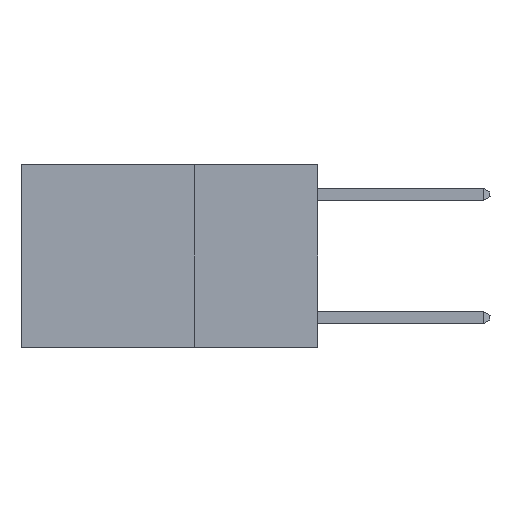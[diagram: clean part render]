
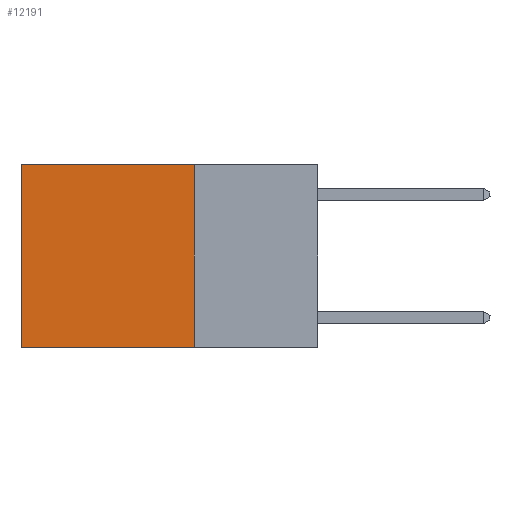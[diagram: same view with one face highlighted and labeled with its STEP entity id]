
A CAD part, left-side view. The second image highlights one B-rep face of the part: STEP entity #12191.
In plain terms, the highlighted planar face has unit normal (-1, 0, 0).
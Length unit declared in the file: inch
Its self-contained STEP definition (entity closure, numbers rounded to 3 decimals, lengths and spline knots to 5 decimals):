
#297 = EDGE_CURVE ( 'NONE', #19565, #20822, #7904, .T. ) ;
#400 = EDGE_CURVE ( 'NONE', #9023, #16624, #6276, .T. ) ;
#967 = DIRECTION ( 'NONE',  ( 0., 0., -1. ) ) ;
#1698 = ORIENTED_EDGE ( 'NONE', *, *, #400, .T. ) ;
#1816 = CARTESIAN_POINT ( 'NONE',  ( 0.2625, 0.25, 0. ) ) ;
#2086 = ORIENTED_EDGE ( 'NONE', *, *, #20383, .T. ) ;
#2225 = VECTOR ( 'NONE', #967, 39.37008 ) ;
#2647 = CARTESIAN_POINT ( 'NONE',  ( 0.2625, 0.6, 0. ) ) ;
#2873 = DIRECTION ( 'NONE',  ( 0., 0., -1. ) ) ;
#4243 = DIRECTION ( 'NONE',  ( 0., 0., -1. ) ) ;
#5708 = EDGE_LOOP ( 'NONE', ( #1698, #7116, #20183, #2086 ) ) ;
#6022 = AXIS2_PLACEMENT_3D ( 'NONE', #8006, #13166, #2873 ) ;
#6276 = LINE ( 'NONE', #2647, #2225 ) ;
#6412 = CARTESIAN_POINT ( 'NONE',  ( 0.2625, 0.25, -0.37 ) ) ;
#7116 = ORIENTED_EDGE ( 'NONE', *, *, #16803, .F. ) ;
#7751 = DIRECTION ( 'NONE',  ( 0., 1., 0. ) ) ;
#7904 = LINE ( 'NONE', #14473, #21235 ) ;
#8006 = CARTESIAN_POINT ( 'NONE',  ( 0.2625, 0.25, 0. ) ) ;
#9023 = VERTEX_POINT ( 'NONE', #10978 ) ;
#10761 = CARTESIAN_POINT ( 'NONE',  ( 0.2625, 0.6, -0.37 ) ) ;
#10978 = CARTESIAN_POINT ( 'NONE',  ( 0.2625, 0.6, 0. ) ) ;
#11438 = PLANE ( 'NONE',  #6022 ) ;
#12136 = VECTOR ( 'NONE', #7751, 39.37008 ) ;
#12191 = ADVANCED_FACE ( 'NONE', ( #19894 ), #11438, .F. ) ;
#13166 = DIRECTION ( 'NONE',  ( 1., 0., 0. ) ) ;
#14473 = CARTESIAN_POINT ( 'NONE',  ( 0.2625, 0.25, 0. ) ) ;
#15269 = VECTOR ( 'NONE', #15477, 39.37008 ) ;
#15477 = DIRECTION ( 'NONE',  ( 0., 1., 0. ) ) ;
#16624 = VERTEX_POINT ( 'NONE', #10761 ) ;
#16803 = EDGE_CURVE ( 'NONE', #20822, #16624, #17066, .T. ) ;
#17066 = LINE ( 'NONE', #19468, #12136 ) ;
#19468 = CARTESIAN_POINT ( 'NONE',  ( 0.2625, 0.25, -0.37 ) ) ;
#19565 = VERTEX_POINT ( 'NONE', #20048 ) ;
#19648 = LINE ( 'NONE', #1816, #15269 ) ;
#19894 = FACE_OUTER_BOUND ( 'NONE', #5708, .T. ) ;
#20048 = CARTESIAN_POINT ( 'NONE',  ( 0.2625, 0.25, 0. ) ) ;
#20183 = ORIENTED_EDGE ( 'NONE', *, *, #297, .F. ) ;
#20383 = EDGE_CURVE ( 'NONE', #19565, #9023, #19648, .T. ) ;
#20822 = VERTEX_POINT ( 'NONE', #6412 ) ;
#21235 = VECTOR ( 'NONE', #4243, 39.37008 ) ;
